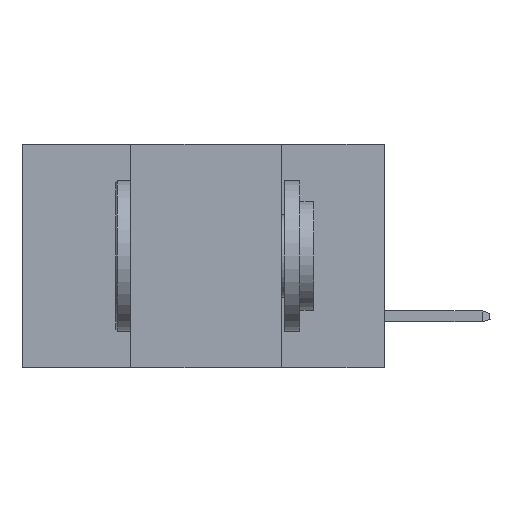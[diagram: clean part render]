
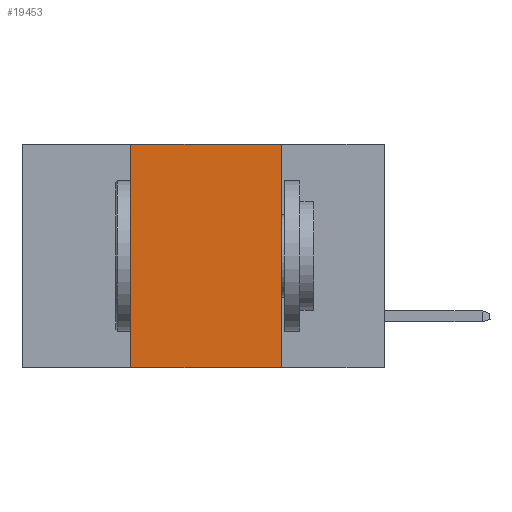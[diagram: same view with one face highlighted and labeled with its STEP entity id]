
A CAD part, left-side view. The second image highlights one B-rep face of the part: STEP entity #19453.
In plain terms, the highlighted planar face has unit normal (-1, 0, 0).
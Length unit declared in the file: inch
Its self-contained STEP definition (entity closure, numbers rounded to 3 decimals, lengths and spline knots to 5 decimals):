
#775 = EDGE_LOOP ( 'NONE', ( #21818, #6103, #22128, #20435 ) ) ;
#2407 = CARTESIAN_POINT ( 'NONE',  ( 0., 0.42, 0. ) ) ;
#2890 = LINE ( 'NONE', #29518, #10419 ) ;
#3144 = PLANE ( 'NONE',  #6420 ) ;
#4547 = DIRECTION ( 'NONE',  ( 0., 0., 1. ) ) ;
#4637 = CARTESIAN_POINT ( 'NONE',  ( 0., 0.17, -0.37 ) ) ;
#6103 = ORIENTED_EDGE ( 'NONE', *, *, #15190, .F. ) ;
#6420 = AXIS2_PLACEMENT_3D ( 'NONE', #8819, #29448, #29250 ) ;
#6883 = EDGE_CURVE ( 'NONE', #22591, #26573, #9788, .T. ) ;
#8819 = CARTESIAN_POINT ( 'NONE',  ( 0., 0.6, 0. ) ) ;
#9054 = DIRECTION ( 'NONE',  ( 0., -1., 0. ) ) ;
#9097 = VERTEX_POINT ( 'NONE', #2407 ) ;
#9329 = CARTESIAN_POINT ( 'NONE',  ( 0., 0.42, -0.37 ) ) ;
#9788 = LINE ( 'NONE', #22681, #22635 ) ;
#10419 = VECTOR ( 'NONE', #18693, 39.37008 ) ;
#11375 = EDGE_CURVE ( 'NONE', #19253, #26573, #24926, .T. ) ;
#14388 = CARTESIAN_POINT ( 'NONE',  ( 0., 0.17, 0. ) ) ;
#15190 = EDGE_CURVE ( 'NONE', #9097, #19253, #2890, .T. ) ;
#16635 = VECTOR ( 'NONE', #4547, 39.37008 ) ;
#18142 = CARTESIAN_POINT ( 'NONE',  ( 0., 0.42, 0. ) ) ;
#18693 = DIRECTION ( 'NONE',  ( 0., -1., 0. ) ) ;
#18847 = DIRECTION ( 'NONE',  ( 0., 0., -1. ) ) ;
#19172 = VECTOR ( 'NONE', #18847, 39.37008 ) ;
#19253 = VERTEX_POINT ( 'NONE', #21857 ) ;
#19453 = ADVANCED_FACE ( 'NONE', ( #27588 ), #3144, .F. ) ;
#20435 = ORIENTED_EDGE ( 'NONE', *, *, #6883, .T. ) ;
#21818 = ORIENTED_EDGE ( 'NONE', *, *, #11375, .F. ) ;
#21857 = CARTESIAN_POINT ( 'NONE',  ( 0., 0.17, 0. ) ) ;
#22128 = ORIENTED_EDGE ( 'NONE', *, *, #25373, .F. ) ;
#22591 = VERTEX_POINT ( 'NONE', #9329 ) ;
#22635 = VECTOR ( 'NONE', #9054, 39.37008 ) ;
#22681 = CARTESIAN_POINT ( 'NONE',  ( 0., 0.6, -0.37 ) ) ;
#24926 = LINE ( 'NONE', #14388, #19172 ) ;
#25373 = EDGE_CURVE ( 'NONE', #22591, #9097, #29536, .T. ) ;
#26573 = VERTEX_POINT ( 'NONE', #4637 ) ;
#27588 = FACE_OUTER_BOUND ( 'NONE', #775, .T. ) ;
#29250 = DIRECTION ( 'NONE',  ( 0., 0., -1. ) ) ;
#29448 = DIRECTION ( 'NONE',  ( 1., 0., 0. ) ) ;
#29518 = CARTESIAN_POINT ( 'NONE',  ( 0., 0.6, 0. ) ) ;
#29536 = LINE ( 'NONE', #18142, #16635 ) ;
